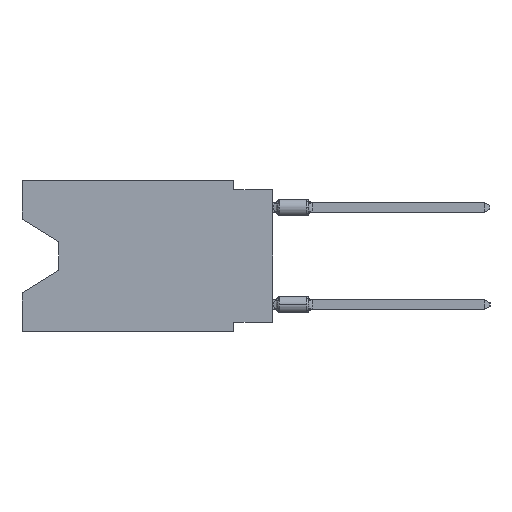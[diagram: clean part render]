
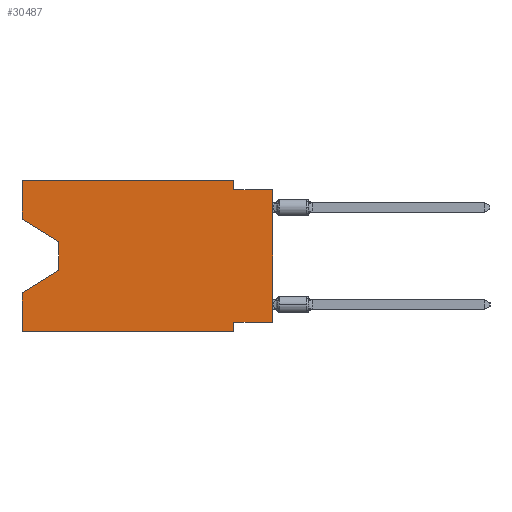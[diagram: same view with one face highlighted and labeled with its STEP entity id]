
A CAD part, left-side view. The second image highlights one B-rep face of the part: STEP entity #30487.
In plain terms, the highlighted planar face has unit normal (-1, 0, 0).
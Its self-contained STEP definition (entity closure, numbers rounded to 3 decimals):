
#217 = FACE_OUTER_BOUND ( 'NONE', #257, .T. ) ;
#257 = EDGE_LOOP ( 'NONE', ( #9360, #39547, #21012, #24961, #40335, #35034, #18977, #18579, #22714, #15687, #42489, #23265 ) ) ;
#1758 = DIRECTION ( 'NONE',  ( 0., 0., -1. ) ) ;
#1879 = LINE ( 'NONE', #9178, #15466 ) ;
#2502 = VERTEX_POINT ( 'NONE', #11172 ) ;
#3439 = VECTOR ( 'NONE', #31203, 1000. ) ;
#4216 = VERTEX_POINT ( 'NONE', #25508 ) ;
#4626 = EDGE_CURVE ( 'NONE', #23908, #33953, #39374, .T. ) ;
#4801 = DIRECTION ( 'NONE',  ( 0., 0., 1. ) ) ;
#5806 = DIRECTION ( 'NONE',  ( 0., 0., -1. ) ) ;
#6749 = EDGE_CURVE ( 'NONE', #36581, #23908, #1879, .T. ) ;
#8981 = EDGE_CURVE ( 'NONE', #15122, #4216, #15876, .T. ) ;
#9178 = CARTESIAN_POINT ( 'NONE',  ( 0., 2.54, 0. ) ) ;
#9230 = VERTEX_POINT ( 'NONE', #29445 ) ;
#9360 = ORIENTED_EDGE ( 'NONE', *, *, #25715, .T. ) ;
#9742 = VECTOR ( 'NONE', #5806, 1000. ) ;
#9747 = LINE ( 'NONE', #13037, #3439 ) ;
#10009 = EDGE_CURVE ( 'NONE', #18725, #39859, #16600, .T. ) ;
#11172 = CARTESIAN_POINT ( 'NONE',  ( 0., 0., -9.271 ) ) ;
#12725 = DIRECTION ( 'NONE',  ( 0., 0., -1. ) ) ;
#13004 = EDGE_CURVE ( 'NONE', #28570, #4216, #29853, .T. ) ;
#13037 = CARTESIAN_POINT ( 'NONE',  ( 0., 16.383, 0. ) ) ;
#14136 = VERTEX_POINT ( 'NONE', #22722 ) ;
#15122 = VERTEX_POINT ( 'NONE', #44778 ) ;
#15466 = VECTOR ( 'NONE', #12725, 1000. ) ;
#15687 = ORIENTED_EDGE ( 'NONE', *, *, #6749, .F. ) ;
#15876 = LINE ( 'NONE', #22488, #43132 ) ;
#16203 = VECTOR ( 'NONE', #29812, 1000. ) ;
#16600 = LINE ( 'NONE', #20137, #17499 ) ;
#16636 = LINE ( 'NONE', #23697, #9742 ) ;
#17416 = LINE ( 'NONE', #39369, #19437 ) ;
#17499 = VECTOR ( 'NONE', #1758, 1000. ) ;
#18130 = DIRECTION ( 'NONE',  ( 0., -1., 0. ) ) ;
#18444 = CARTESIAN_POINT ( 'NONE',  ( 0., 2.54, -0.635 ) ) ;
#18579 = ORIENTED_EDGE ( 'NONE', *, *, #45958, .T. ) ;
#18725 = VERTEX_POINT ( 'NONE', #30216 ) ;
#18977 = ORIENTED_EDGE ( 'NONE', *, *, #27173, .F. ) ;
#19293 = VECTOR ( 'NONE', #33925, 1000. ) ;
#19437 = VECTOR ( 'NONE', #31809, 1000. ) ;
#19538 = LINE ( 'NONE', #27303, #19293 ) ;
#20137 = CARTESIAN_POINT ( 'NONE',  ( 0., 2.54, -9.906 ) ) ;
#20853 = VECTOR ( 'NONE', #28286, 1000. ) ;
#21012 = ORIENTED_EDGE ( 'NONE', *, *, #13004, .T. ) ;
#21196 = DIRECTION ( 'NONE',  ( 0., 0., -1. ) ) ;
#22488 = CARTESIAN_POINT ( 'NONE',  ( 0., 16.383, 0. ) ) ;
#22714 = ORIENTED_EDGE ( 'NONE', *, *, #4626, .F. ) ;
#22722 = CARTESIAN_POINT ( 'NONE',  ( 0., 13.97, -4.013 ) ) ;
#23265 = ORIENTED_EDGE ( 'NONE', *, *, #23572, .F. ) ;
#23380 = EDGE_CURVE ( 'NONE', #15122, #39859, #44665, .T. ) ;
#23572 = EDGE_CURVE ( 'NONE', #9230, #35076, #9747, .T. ) ;
#23697 = CARTESIAN_POINT ( 'NONE',  ( 0., 13.97, -4.013 ) ) ;
#23908 = VERTEX_POINT ( 'NONE', #18444 ) ;
#24384 = EDGE_CURVE ( 'NONE', #35076, #36581, #19538, .T. ) ;
#24748 = PLANE ( 'NONE',  #24767 ) ;
#24767 = AXIS2_PLACEMENT_3D ( 'NONE', #31820, #46213, #21196 ) ;
#24961 = ORIENTED_EDGE ( 'NONE', *, *, #8981, .F. ) ;
#25508 = CARTESIAN_POINT ( 'NONE',  ( 0., 16.383, -7.36 ) ) ;
#25715 = EDGE_CURVE ( 'NONE', #9230, #14136, #35601, .T. ) ;
#25727 = VECTOR ( 'NONE', #39699, 1000. ) ;
#27173 = EDGE_CURVE ( 'NONE', #2502, #18725, #28822, .T. ) ;
#27303 = CARTESIAN_POINT ( 'NONE',  ( 0., 16.383, 0. ) ) ;
#28286 = DIRECTION ( 'NONE',  ( 0., -0.855, -0.519 ) ) ;
#28570 = VERTEX_POINT ( 'NONE', #33979 ) ;
#28822 = LINE ( 'NONE', #43229, #25727 ) ;
#29441 = CARTESIAN_POINT ( 'NONE',  ( 0., 16.383, 0. ) ) ;
#29445 = CARTESIAN_POINT ( 'NONE',  ( 0., 16.383, -2.546 ) ) ;
#29812 = DIRECTION ( 'NONE',  ( 0., -1., 0. ) ) ;
#29853 = LINE ( 'NONE', #37150, #32741 ) ;
#30216 = CARTESIAN_POINT ( 'NONE',  ( 0., 2.54, -9.271 ) ) ;
#30487 = ADVANCED_FACE ( 'NONE', ( #217 ), #24748, .F. ) ;
#31203 = DIRECTION ( 'NONE',  ( 0., 0., 1. ) ) ;
#31809 = DIRECTION ( 'NONE',  ( 0., 0., 1. ) ) ;
#31820 = CARTESIAN_POINT ( 'NONE',  ( 0., 16.383, 0. ) ) ;
#32741 = VECTOR ( 'NONE', #44255, 1000. ) ;
#33925 = DIRECTION ( 'NONE',  ( 0., -1., 0. ) ) ;
#33953 = VERTEX_POINT ( 'NONE', #34066 ) ;
#33979 = CARTESIAN_POINT ( 'NONE',  ( 0., 13.97, -5.893 ) ) ;
#34040 = CARTESIAN_POINT ( 'NONE',  ( 0., 16.383, -9.906 ) ) ;
#34066 = CARTESIAN_POINT ( 'NONE',  ( 0., 0., -0.635 ) ) ;
#35034 = ORIENTED_EDGE ( 'NONE', *, *, #10009, .F. ) ;
#35076 = VERTEX_POINT ( 'NONE', #29441 ) ;
#35601 = LINE ( 'NONE', #39390, #20853 ) ;
#36311 = VECTOR ( 'NONE', #18130, 1000. ) ;
#36581 = VERTEX_POINT ( 'NONE', #39338 ) ;
#37150 = CARTESIAN_POINT ( 'NONE',  ( 0., 13.97, -5.893 ) ) ;
#39077 = EDGE_CURVE ( 'NONE', #14136, #28570, #16636, .T. ) ;
#39338 = CARTESIAN_POINT ( 'NONE',  ( 0., 2.54, 0. ) ) ;
#39369 = CARTESIAN_POINT ( 'NONE',  ( 0., 0., 0. ) ) ;
#39374 = LINE ( 'NONE', #39850, #36311 ) ;
#39390 = CARTESIAN_POINT ( 'NONE',  ( 0., 16.383, -2.546 ) ) ;
#39547 = ORIENTED_EDGE ( 'NONE', *, *, #39077, .T. ) ;
#39699 = DIRECTION ( 'NONE',  ( 0., 1., 0. ) ) ;
#39850 = CARTESIAN_POINT ( 'NONE',  ( 0., 0., -0.635 ) ) ;
#39859 = VERTEX_POINT ( 'NONE', #42424 ) ;
#40335 = ORIENTED_EDGE ( 'NONE', *, *, #23380, .T. ) ;
#42424 = CARTESIAN_POINT ( 'NONE',  ( 0., 2.54, -9.906 ) ) ;
#42489 = ORIENTED_EDGE ( 'NONE', *, *, #24384, .F. ) ;
#43132 = VECTOR ( 'NONE', #4801, 1000. ) ;
#43229 = CARTESIAN_POINT ( 'NONE',  ( 0., 0., -9.271 ) ) ;
#44255 = DIRECTION ( 'NONE',  ( 0., 0.855, -0.519 ) ) ;
#44665 = LINE ( 'NONE', #34040, #16203 ) ;
#44778 = CARTESIAN_POINT ( 'NONE',  ( 0., 16.383, -9.906 ) ) ;
#45958 = EDGE_CURVE ( 'NONE', #2502, #33953, #17416, .T. ) ;
#46213 = DIRECTION ( 'NONE',  ( 1., 0., 0. ) ) ;
